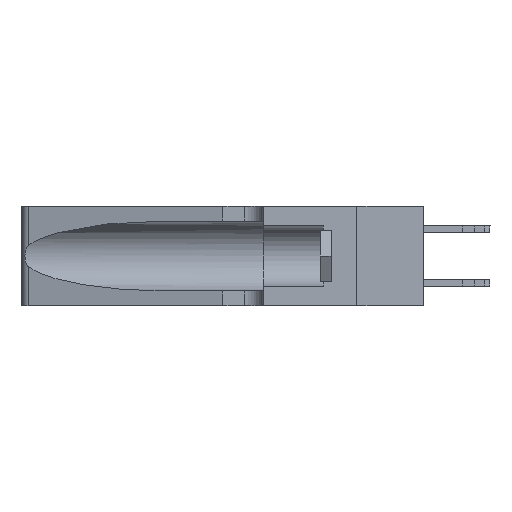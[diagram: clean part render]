
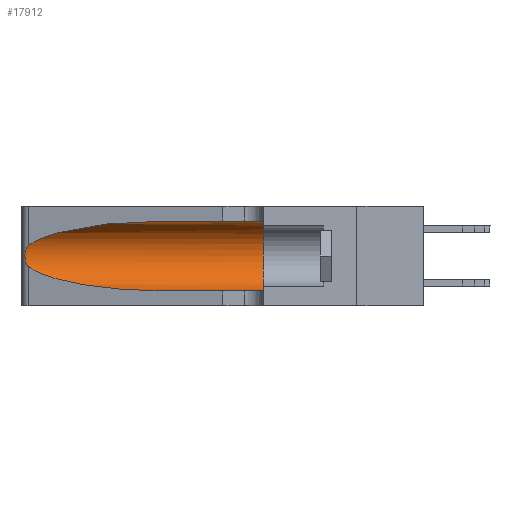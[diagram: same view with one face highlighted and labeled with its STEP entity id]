
A CAD part, left-side view. The second image highlights one B-rep face of the part: STEP entity #17912.
In plain terms, the highlighted cylindrical face has radius 3.308 mm (diameter 6.617 mm), a partial arc.
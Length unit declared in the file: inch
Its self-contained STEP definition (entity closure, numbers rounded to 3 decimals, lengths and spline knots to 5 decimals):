
#205 = LINE ( 'NONE', #13423, #17575 ) ;
#883 = CARTESIAN_POINT ( 'NONE',  ( 0.1305, 0.72297, 0.05475 ) ) ;
#1008 = CARTESIAN_POINT ( 'NONE',  ( 0.1305, 0.35, 0.185 ) ) ;
#1384 = EDGE_CURVE ( 'NONE', #18661, #21995, #23122, .T. ) ;
#1486 = CARTESIAN_POINT ( 'NONE',  ( 0.1305, 0.72297, 0.05475 ) ) ;
#1563 = CARTESIAN_POINT ( 'NONE',  ( 0.26075, 1.23896, 0.178 ) ) ;
#1907 = EDGE_CURVE ( 'NONE', #18108, #2224, #20231, .T. ) ;
#1918 = CARTESIAN_POINT ( 'NONE',  ( 0.26075, 1.23896, 0.19203 ) ) ;
#1949 = CARTESIAN_POINT ( 'NONE',  ( 0.1305, 0.72297, 0.31525 ) ) ;
#2224 = VERTEX_POINT ( 'NONE', #1486 ) ;
#2676 = EDGE_CURVE ( 'NONE', #2224, #14453, #205, .T. ) ;
#3926 = CARTESIAN_POINT ( 'NONE',  ( 0.25854, 1.2359, 0.20912 ) ) ;
#4349 = EDGE_CURVE ( 'NONE', #21995, #18108, #17678, .T. ) ;
#6619 = VERTEX_POINT ( 'NONE', #14602 ) ;
#7107 = DIRECTION ( 'NONE',  ( 0., -1., 0. ) ) ;
#8063 = CARTESIAN_POINT ( 'NONE',  ( 0.18966, 0.96281, 0.31525 ) ) ;
#8391 = CARTESIAN_POINT ( 'NONE',  ( 0.25487, 1.22718, 0.14631 ) ) ;
#8475 = CARTESIAN_POINT ( 'NONE',  ( 0.25789, 1.23486, 0.15765 ) ) ;
#8715 = EDGE_LOOP ( 'NONE', ( #18750, #25729, #19979, #23004, #25524, #26249 ) ) ;
#9661 = AXIS2_PLACEMENT_3D ( 'NONE', #12398, #12482, #16783 ) ;
#10064 = CARTESIAN_POINT ( 'NONE',  ( 0.25487, 1.22718, 0.22369 ) ) ;
#10389 = CARTESIAN_POINT ( 'NONE',  ( 0.1305, 0.35, 0.05475 ) ) ;
#10963 = LINE ( 'NONE', #22008, #16168 ) ;
#11677 = CARTESIAN_POINT ( 'NONE',  ( 0.18966, 0.96281, 0.05475 ) ) ;
#11987 = CARTESIAN_POINT ( 'NONE',  ( 0.25555, 1.22994, 0.2215 ) ) ;
#12398 = CARTESIAN_POINT ( 'NONE',  ( 0.1305, 1.61858, 0.185 ) ) ;
#12482 = DIRECTION ( 'NONE',  ( 0., -1., 0. ) ) ;
#13423 = CARTESIAN_POINT ( 'NONE',  ( 0.1305, 1.61858, 0.05475 ) ) ;
#14202 = CARTESIAN_POINT ( 'NONE',  ( 0.25487, 1.22718, 0.22369 ) ) ;
#14453 = VERTEX_POINT ( 'NONE', #10389 ) ;
#14602 = CARTESIAN_POINT ( 'NONE',  ( 0.1305, 0.35, 0.31525 ) ) ;
#14690 = CARTESIAN_POINT ( 'NONE',  ( 0.25555, 1.22993, 0.14849 ) ) ;
#15316 = EDGE_CURVE ( 'NONE', #6619, #14453, #19511, .T. ) ;
#15614 = DIRECTION ( 'NONE',  ( 0., 1., 0. ) ) ;
#16165 = CARTESIAN_POINT ( 'NONE',  ( 0.26017, 1.23833, 0.17102 ) ) ;
#16168 = VECTOR ( 'NONE', #7107, 39.37008 ) ;
#16441 = CARTESIAN_POINT ( 'NONE',  ( 0.25639, 1.23184, 0.21858 ) ) ;
#16541 = CARTESIAN_POINT ( 'NONE',  ( 0.25856, 1.23593, 0.16098 ) ) ;
#16783 = DIRECTION ( 'NONE',  ( 0., 0., -1. ) ) ;
#17575 = VECTOR ( 'NONE', #21838, 39.37008 ) ;
#17639 = DIRECTION ( 'NONE',  ( 0., 0., 1. ) ) ;
#17678 = B_SPLINE_CURVE_WITH_KNOTS ( 'NONE', 3,
 ( #10064, #11987, #16441, #26758, #3926, #24963, #1918, #1563, #16165, #16541, #8475, #20978, #14690, #8391 ),
 .UNSPECIFIED., .F., .F.,
 ( 4, 2, 2, 2, 2, 2, 4 ),
 ( 0., 0.00027, 0.00053, 0.00107, 0.0016, 0.00187, 0.00214 ),
 .UNSPECIFIED. ) ;
#17912 = ADVANCED_FACE ( 'NONE', ( #24659 ), #18996, .F. ) ;
#18108 = VERTEX_POINT ( 'NONE', #21321 ) ;
#18661 = VERTEX_POINT ( 'NONE', #1949 ) ;
#18750 = ORIENTED_EDGE ( 'NONE', *, *, #1384, .T. ) ;
#18996 = CYLINDRICAL_SURFACE ( 'NONE', #9661, 0.13025 ) ;
#19511 = CIRCLE ( 'NONE', #25521, 0.13025 ) ;
#19919 = CARTESIAN_POINT ( 'NONE',  ( 0.25487, 1.22718, 0.14631 ) ) ;
#19979 = ORIENTED_EDGE ( 'NONE', *, *, #1907, .T. ) ;
#20175 = CARTESIAN_POINT ( 'NONE',  ( 0.1305, 0.72297, 0.31525 ) ) ;
#20231 =( BOUNDED_CURVE ( )  B_SPLINE_CURVE ( 3, ( #19919, #24187, #11677, #883 ),
 .UNSPECIFIED., .F., .F. ) 
 B_SPLINE_CURVE_WITH_KNOTS ( ( 4, 4 ),
 ( 3.44316, 4.71239 ),
 .UNSPECIFIED. ) 
 CURVE ( )  GEOMETRIC_REPRESENTATION_ITEM ( )  RATIONAL_B_SPLINE_CURVE ( ( 1., 0.87, 0.87, 1. ) ) 
 REPRESENTATION_ITEM ( '' )  );
#20636 = CARTESIAN_POINT ( 'NONE',  ( 0.2373, 1.15595, 0.28018 ) ) ;
#20978 = CARTESIAN_POINT ( 'NONE',  ( 0.25639, 1.23186, 0.15144 ) ) ;
#21321 = CARTESIAN_POINT ( 'NONE',  ( 0.25487, 1.22718, 0.14631 ) ) ;
#21838 = DIRECTION ( 'NONE',  ( 0., -1., 0. ) ) ;
#21995 = VERTEX_POINT ( 'NONE', #26044 ) ;
#22008 = CARTESIAN_POINT ( 'NONE',  ( 0.1305, 1.61858, 0.31525 ) ) ;
#23004 = ORIENTED_EDGE ( 'NONE', *, *, #2676, .T. ) ;
#23122 =( BOUNDED_CURVE ( )  B_SPLINE_CURVE ( 3, ( #20175, #8063, #20636, #14202 ),
 .UNSPECIFIED., .F., .F. ) 
 B_SPLINE_CURVE_WITH_KNOTS ( ( 4, 4 ),
 ( 1.5708, 2.84003 ),
 .UNSPECIFIED. ) 
 CURVE ( )  GEOMETRIC_REPRESENTATION_ITEM ( )  RATIONAL_B_SPLINE_CURVE ( ( 1., 0.87, 0.87, 1. ) ) 
 REPRESENTATION_ITEM ( '' )  );
#23170 = EDGE_CURVE ( 'NONE', #18661, #6619, #10963, .T. ) ;
#24187 = CARTESIAN_POINT ( 'NONE',  ( 0.2373, 1.15595, 0.08982 ) ) ;
#24659 = FACE_OUTER_BOUND ( 'NONE', #8715, .T. ) ;
#24963 = CARTESIAN_POINT ( 'NONE',  ( 0.26018, 1.23835, 0.19895 ) ) ;
#25521 = AXIS2_PLACEMENT_3D ( 'NONE', #1008, #15614, #17639 ) ;
#25524 = ORIENTED_EDGE ( 'NONE', *, *, #15316, .F. ) ;
#25729 = ORIENTED_EDGE ( 'NONE', *, *, #4349, .T. ) ;
#26044 = CARTESIAN_POINT ( 'NONE',  ( 0.25487, 1.22718, 0.22369 ) ) ;
#26249 = ORIENTED_EDGE ( 'NONE', *, *, #23170, .F. ) ;
#26758 = CARTESIAN_POINT ( 'NONE',  ( 0.25787, 1.23484, 0.2124 ) ) ;
